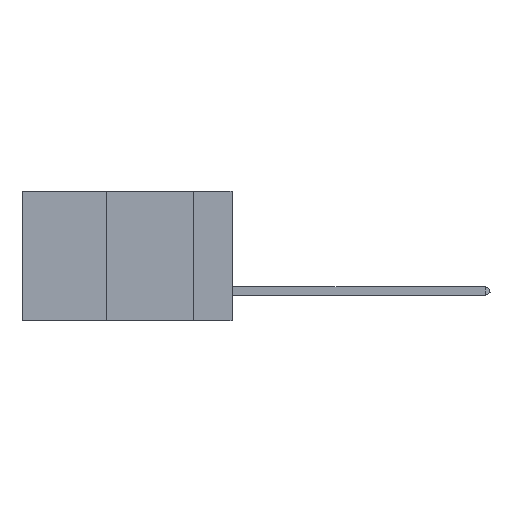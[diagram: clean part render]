
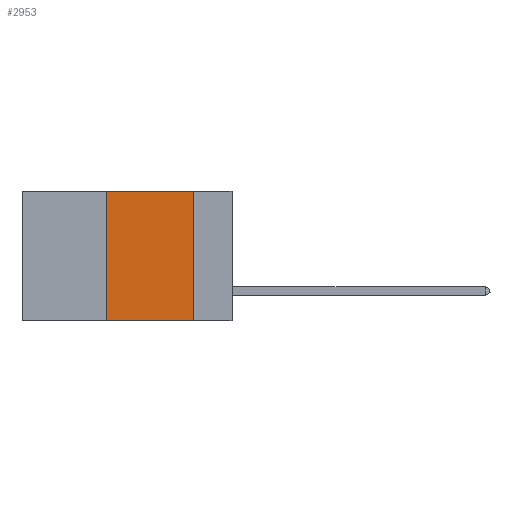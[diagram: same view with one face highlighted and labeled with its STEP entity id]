
A CAD part, left-side view. The second image highlights one B-rep face of the part: STEP entity #2953.
In plain terms, the highlighted planar face has unit normal (-1, 0, 0).
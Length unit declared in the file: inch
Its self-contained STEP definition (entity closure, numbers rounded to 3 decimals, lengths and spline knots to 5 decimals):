
#806 = EDGE_CURVE ( 'NONE', #1956, #15796, #7122, .T. ) ;
#936 = VECTOR ( 'NONE', #5866, 39.37008 ) ;
#1454 = EDGE_CURVE ( 'NONE', #15796, #14277, #19261, .T. ) ;
#1956 = VERTEX_POINT ( 'NONE', #6769 ) ;
#2298 = PLANE ( 'NONE',  #5353 ) ;
#2638 = DIRECTION ( 'NONE',  ( 0., -1., 0. ) ) ;
#2953 = ADVANCED_FACE ( 'NONE', ( #19611 ), #2298, .F. ) ;
#3467 = CARTESIAN_POINT ( 'NONE',  ( 0., 0.6, -0.37 ) ) ;
#3652 = ORIENTED_EDGE ( 'NONE', *, *, #10327, .T. ) ;
#3887 = VECTOR ( 'NONE', #2638, 39.37008 ) ;
#5290 = ORIENTED_EDGE ( 'NONE', *, *, #806, .F. ) ;
#5353 = AXIS2_PLACEMENT_3D ( 'NONE', #21478, #21255, #12700 ) ;
#5866 = DIRECTION ( 'NONE',  ( 0., 0., -1. ) ) ;
#6769 = CARTESIAN_POINT ( 'NONE',  ( 0., 0.36, -0.37 ) ) ;
#7122 = LINE ( 'NONE', #16609, #10660 ) ;
#7930 = CARTESIAN_POINT ( 'NONE',  ( 0., 0.11, 0. ) ) ;
#10327 = EDGE_CURVE ( 'NONE', #1956, #21732, #13906, .T. ) ;
#10660 = VECTOR ( 'NONE', #16358, 39.37008 ) ;
#11159 = LINE ( 'NONE', #14578, #936 ) ;
#11264 = ORIENTED_EDGE ( 'NONE', *, *, #18104, .F. ) ;
#12059 = CARTESIAN_POINT ( 'NONE',  ( 0., 0.11, -0.37 ) ) ;
#12700 = DIRECTION ( 'NONE',  ( 0., 0., -1. ) ) ;
#12807 = CARTESIAN_POINT ( 'NONE',  ( 0., 0.6, 0. ) ) ;
#13906 = LINE ( 'NONE', #3467, #19539 ) ;
#14277 = VERTEX_POINT ( 'NONE', #7930 ) ;
#14578 = CARTESIAN_POINT ( 'NONE',  ( 0., 0.11, 0. ) ) ;
#15796 = VERTEX_POINT ( 'NONE', #15852 ) ;
#15852 = CARTESIAN_POINT ( 'NONE',  ( 0., 0.36, 0. ) ) ;
#16358 = DIRECTION ( 'NONE',  ( 0., 0., 1. ) ) ;
#16609 = CARTESIAN_POINT ( 'NONE',  ( 0., 0.36, 0. ) ) ;
#17313 = DIRECTION ( 'NONE',  ( 0., -1., 0. ) ) ;
#18104 = EDGE_CURVE ( 'NONE', #14277, #21732, #11159, .T. ) ;
#19195 = ORIENTED_EDGE ( 'NONE', *, *, #1454, .F. ) ;
#19261 = LINE ( 'NONE', #12807, #3887 ) ;
#19539 = VECTOR ( 'NONE', #17313, 39.37008 ) ;
#19611 = FACE_OUTER_BOUND ( 'NONE', #19644, .T. ) ;
#19644 = EDGE_LOOP ( 'NONE', ( #11264, #19195, #5290, #3652 ) ) ;
#21255 = DIRECTION ( 'NONE',  ( 1., 0., 0. ) ) ;
#21478 = CARTESIAN_POINT ( 'NONE',  ( 0., 0.6, 0. ) ) ;
#21732 = VERTEX_POINT ( 'NONE', #12059 ) ;
